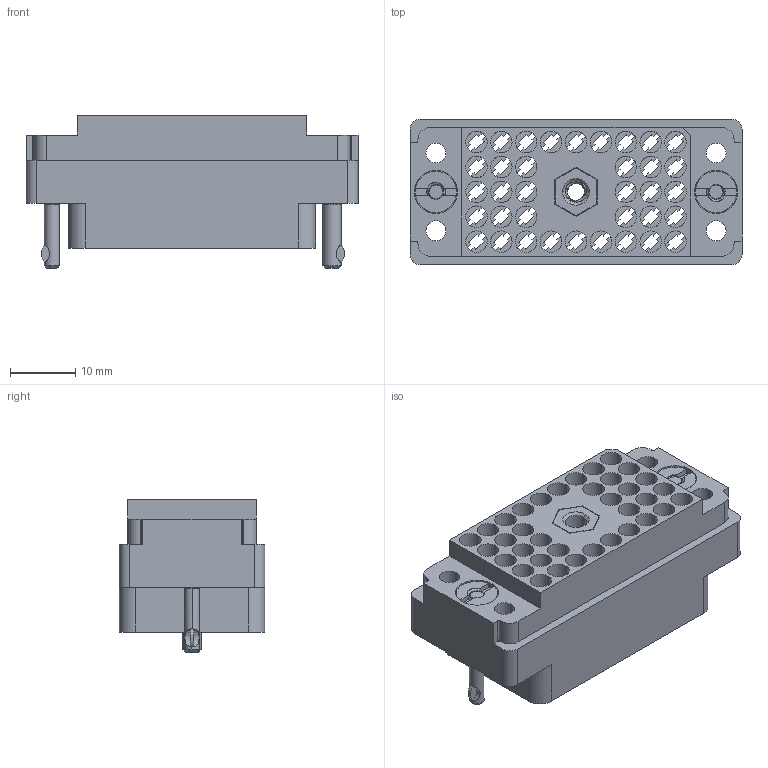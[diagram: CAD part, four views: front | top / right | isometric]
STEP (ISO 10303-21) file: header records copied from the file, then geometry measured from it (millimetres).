
FILE_DESCRIPTION (( 'STEP AP203' ), '1' );
FILE_NAME ('519-036-000-302.STEP', '2020-03-11T16:02:02', ( '' ), ( '' ), 'SwSTEP 2.0', 'SolidWorks 2016', '' );
FILE_SCHEMA (( 'CONFIG_CONTROL_DESIGN' ));
Length unit declared in the file: inch
Products named in the file (6): 519 Plug Insulator_036; 519-036-000-302; 516-222-038-102_038; 516-252-021-102_038; 516-222-038-102_039; 516-252-035-100_516-252-035-100
Assembly tree (6 placements, depth 2):
  519-036-000-302
    519 Plug Insulator_036
    516-252-035-100_516-252-035-100
    516-252-021-102_038  x2
    516-222-038-102_038
    516-222-038-102_039
Bounding box: 50.8 x 22.25 x 23.37 mm (x, y, z)
Volume: 9524.5 mm3; surface area: 12535 mm2
Topology: 6 solids, 6 shells, 1092 faces, 3111 edges, 2054 vertices
Faces by surface type: plane 670, cylinder 330, cone 46, bspline 42, torus 4
Entity records: 41894 total; most frequent: CARTESIAN_POINT 13332, ORIENTED_EDGE 6042, DIRECTION 5637, EDGE_CURVE 3021, LINE 2029, VECTOR 2029, VERTEX_POINT 1994, AXIS2_PLACEMENT_3D 1804
